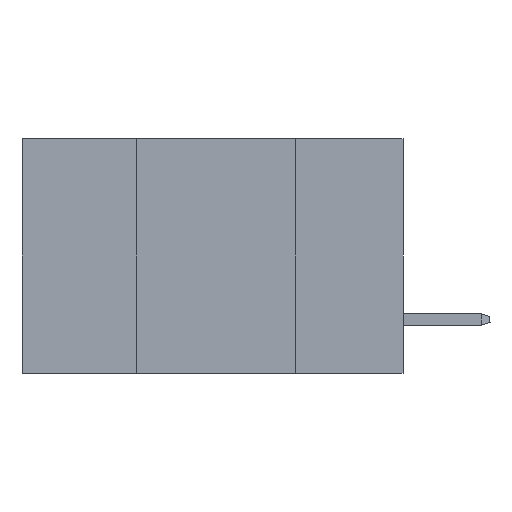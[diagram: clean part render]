
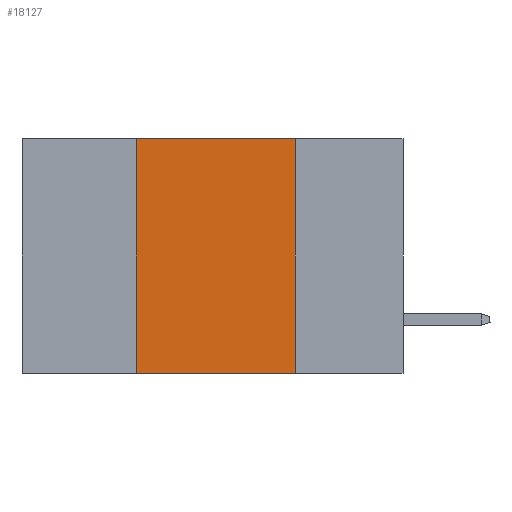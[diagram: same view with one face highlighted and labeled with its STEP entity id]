
A CAD part, left-side view. The second image highlights one B-rep face of the part: STEP entity #18127.
In plain terms, the highlighted planar face has unit normal (-1, 0, 0).
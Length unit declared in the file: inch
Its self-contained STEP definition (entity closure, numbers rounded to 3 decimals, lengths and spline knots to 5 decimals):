
#448 = VERTEX_POINT ( 'NONE', #32840 ) ;
#776 = VECTOR ( 'NONE', #13459, 39.37008 ) ;
#1849 = CARTESIAN_POINT ( 'NONE',  ( 0., 0.17, 0. ) ) ;
#3140 = VECTOR ( 'NONE', #10025, 39.37008 ) ;
#5712 = EDGE_CURVE ( 'NONE', #448, #30499, #31506, .T. ) ;
#6762 = DIRECTION ( 'NONE',  ( 1., 0., 0. ) ) ;
#8355 = FACE_OUTER_BOUND ( 'NONE', #44301, .T. ) ;
#8782 = CARTESIAN_POINT ( 'NONE',  ( 0., 0.42, 0. ) ) ;
#9176 = LINE ( 'NONE', #20380, #776 ) ;
#10025 = DIRECTION ( 'NONE',  ( 0., -1., 0. ) ) ;
#13459 = DIRECTION ( 'NONE',  ( 0., 0., 1. ) ) ;
#14380 = PLANE ( 'NONE',  #40649 ) ;
#14851 = CARTESIAN_POINT ( 'NONE',  ( 0., 0.6, 0. ) ) ;
#16719 = LINE ( 'NONE', #39863, #42469 ) ;
#17629 = ORIENTED_EDGE ( 'NONE', *, *, #39718, .F. ) ;
#17936 = ORIENTED_EDGE ( 'NONE', *, *, #36905, .F. ) ;
#18127 = ADVANCED_FACE ( 'NONE', ( #8355 ), #14380, .F. ) ;
#20380 = CARTESIAN_POINT ( 'NONE',  ( 0., 0.42, 0. ) ) ;
#24887 = DIRECTION ( 'NONE',  ( 0., 0., -1. ) ) ;
#27459 = ORIENTED_EDGE ( 'NONE', *, *, #46923, .F. ) ;
#28859 = CARTESIAN_POINT ( 'NONE',  ( 0., 0.6, -0.37 ) ) ;
#30499 = VERTEX_POINT ( 'NONE', #39442 ) ;
#31174 = VERTEX_POINT ( 'NONE', #1849 ) ;
#31238 = VERTEX_POINT ( 'NONE', #8782 ) ;
#31506 = LINE ( 'NONE', #28859, #3140 ) ;
#32840 = CARTESIAN_POINT ( 'NONE',  ( 0., 0.42, -0.37 ) ) ;
#35837 = CARTESIAN_POINT ( 'NONE',  ( 0., 0.6, 0. ) ) ;
#36905 = EDGE_CURVE ( 'NONE', #448, #31238, #9176, .T. ) ;
#38604 = ORIENTED_EDGE ( 'NONE', *, *, #5712, .T. ) ;
#39442 = CARTESIAN_POINT ( 'NONE',  ( 0., 0.17, -0.37 ) ) ;
#39639 = DIRECTION ( 'NONE',  ( 0., 0., -1. ) ) ;
#39718 = EDGE_CURVE ( 'NONE', #31238, #31174, #46381, .T. ) ;
#39863 = CARTESIAN_POINT ( 'NONE',  ( 0., 0.17, 0. ) ) ;
#40649 = AXIS2_PLACEMENT_3D ( 'NONE', #14851, #6762, #24887 ) ;
#42469 = VECTOR ( 'NONE', #39639, 39.37008 ) ;
#44301 = EDGE_LOOP ( 'NONE', ( #27459, #17629, #17936, #38604 ) ) ;
#45416 = VECTOR ( 'NONE', #46613, 39.37008 ) ;
#46381 = LINE ( 'NONE', #35837, #45416 ) ;
#46613 = DIRECTION ( 'NONE',  ( 0., -1., 0. ) ) ;
#46923 = EDGE_CURVE ( 'NONE', #31174, #30499, #16719, .T. ) ;
